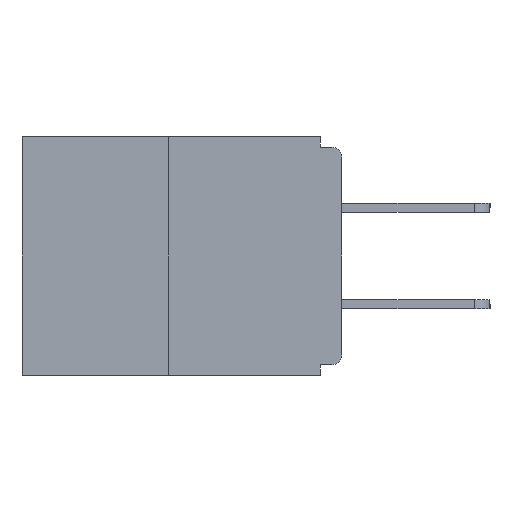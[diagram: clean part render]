
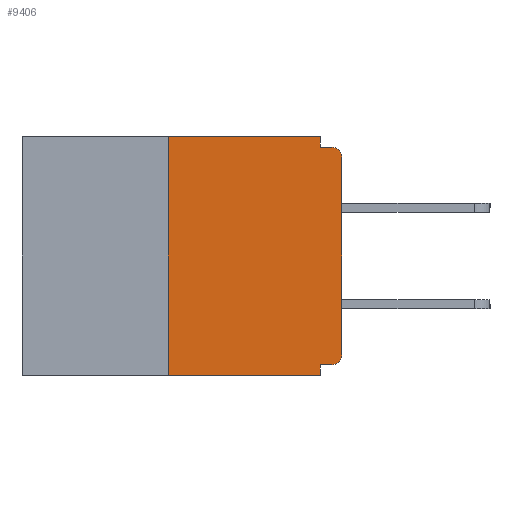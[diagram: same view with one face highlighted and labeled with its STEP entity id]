
A CAD part, left-side view. The second image highlights one B-rep face of the part: STEP entity #9406.
In plain terms, the highlighted planar face has unit normal (-1, 0, 0).
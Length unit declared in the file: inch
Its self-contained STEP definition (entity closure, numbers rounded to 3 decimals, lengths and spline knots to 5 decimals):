
#80 = VERTEX_POINT ( 'NONE', #13878 ) ;
#172 = VERTEX_POINT ( 'NONE', #8825 ) ;
#313 = CARTESIAN_POINT ( 'NONE',  ( 0., 0.015, -0.313 ) ) ;
#504 = LINE ( 'NONE', #13749, #7984 ) ;
#730 = EDGE_CURVE ( 'NONE', #14701, #11607, #9278, .T. ) ;
#771 = LINE ( 'NONE', #9872, #14488 ) ;
#1022 = VECTOR ( 'NONE', #3126, 39.37008 ) ;
#1107 = VERTEX_POINT ( 'NONE', #13405 ) ;
#1111 = AXIS2_PLACEMENT_3D ( 'NONE', #313, #15336, #6957 ) ;
#1168 = CARTESIAN_POINT ( 'NONE',  ( 0., 0., 0. ) ) ;
#1412 = CARTESIAN_POINT ( 'NONE',  ( 0., 0.015, -0.328 ) ) ;
#1575 = CARTESIAN_POINT ( 'NONE',  ( 0., 0.46, -0.343 ) ) ;
#1617 = DIRECTION ( 'NONE',  ( 1., 0., 0. ) ) ;
#1954 = ORIENTED_EDGE ( 'NONE', *, *, #13852, .F. ) ;
#2118 = EDGE_CURVE ( 'NONE', #15486, #172, #3852, .T. ) ;
#2410 = DIRECTION ( 'NONE',  ( 0., 0., 1. ) ) ;
#2470 = VECTOR ( 'NONE', #14246, 39.37008 ) ;
#3126 = DIRECTION ( 'NONE',  ( 0., 0., -1. ) ) ;
#3182 = CARTESIAN_POINT ( 'NONE',  ( 0., 0.031, 0. ) ) ;
#3269 = EDGE_CURVE ( 'NONE', #80, #11607, #504, .T. ) ;
#3852 = LINE ( 'NONE', #15900, #9210 ) ;
#4081 = VECTOR ( 'NONE', #6860, 39.37008 ) ;
#5184 = ORIENTED_EDGE ( 'NONE', *, *, #7156, .T. ) ;
#5277 = CARTESIAN_POINT ( 'NONE',  ( 0., 0.015, -0.03 ) ) ;
#6860 = DIRECTION ( 'NONE',  ( 0., -1., 0. ) ) ;
#6922 = EDGE_CURVE ( 'NONE', #14485, #11233, #11307, .T. ) ;
#6957 = DIRECTION ( 'NONE',  ( 0., 0., -1. ) ) ;
#7137 = AXIS2_PLACEMENT_3D ( 'NONE', #8317, #1617, #16765 ) ;
#7156 = EDGE_CURVE ( 'NONE', #1107, #14701, #9352, .T. ) ;
#7200 = ORIENTED_EDGE ( 'NONE', *, *, #6922, .F. ) ;
#7305 = CARTESIAN_POINT ( 'NONE',  ( 0., 0.015, -0.015 ) ) ;
#7648 = CIRCLE ( 'NONE', #1111, 0.015 ) ;
#7684 = CARTESIAN_POINT ( 'NONE',  ( 0., 0.031, -0.343 ) ) ;
#7907 = DIRECTION ( 'NONE',  ( 0., 0., -1. ) ) ;
#7984 = VECTOR ( 'NONE', #8351, 39.37008 ) ;
#8054 = EDGE_CURVE ( 'NONE', #11233, #14137, #771, .T. ) ;
#8214 = EDGE_CURVE ( 'NONE', #172, #8375, #12112, .T. ) ;
#8317 = CARTESIAN_POINT ( 'NONE',  ( 0., 0.46, 0. ) ) ;
#8351 = DIRECTION ( 'NONE',  ( 0., -1., 0. ) ) ;
#8375 = VERTEX_POINT ( 'NONE', #7684 ) ;
#8595 = LINE ( 'NONE', #1575, #4081 ) ;
#8604 = DIRECTION ( 'NONE',  ( 0., -1., 0. ) ) ;
#8675 = ORIENTED_EDGE ( 'NONE', *, *, #3269, .F. ) ;
#8825 = CARTESIAN_POINT ( 'NONE',  ( 0., 0.031, -0.328 ) ) ;
#8828 = EDGE_CURVE ( 'NONE', #14485, #8375, #8595, .T. ) ;
#9210 = VECTOR ( 'NONE', #10452, 39.37008 ) ;
#9224 = DIRECTION ( 'NONE',  ( -1., 0., 0. ) ) ;
#9278 = CIRCLE ( 'NONE', #13974, 0.015 ) ;
#9352 = LINE ( 'NONE', #1168, #12998 ) ;
#9406 = ADVANCED_FACE ( 'NONE', ( #16803 ), #16652, .F. ) ;
#9797 = LINE ( 'NONE', #3182, #1022 ) ;
#9872 = CARTESIAN_POINT ( 'NONE',  ( 0., 0.46, 0. ) ) ;
#10452 = DIRECTION ( 'NONE',  ( 0., 1., 0. ) ) ;
#10947 = DIRECTION ( 'NONE',  ( 0., 0., 1. ) ) ;
#11212 = ORIENTED_EDGE ( 'NONE', *, *, #730, .T. ) ;
#11233 = VERTEX_POINT ( 'NONE', #13191 ) ;
#11307 = LINE ( 'NONE', #11829, #14946 ) ;
#11607 = VERTEX_POINT ( 'NONE', #7305 ) ;
#11829 = CARTESIAN_POINT ( 'NONE',  ( 0., 0.25, 0. ) ) ;
#11855 = ORIENTED_EDGE ( 'NONE', *, *, #8828, .T. ) ;
#12112 = LINE ( 'NONE', #14357, #2470 ) ;
#12998 = VECTOR ( 'NONE', #10947, 39.37008 ) ;
#13191 = CARTESIAN_POINT ( 'NONE',  ( 0., 0.25, 0. ) ) ;
#13405 = CARTESIAN_POINT ( 'NONE',  ( 0., 0., -0.313 ) ) ;
#13526 = EDGE_CURVE ( 'NONE', #15486, #1107, #7648, .T. ) ;
#13531 = CARTESIAN_POINT ( 'NONE',  ( 0., 0.031, 0. ) ) ;
#13749 = CARTESIAN_POINT ( 'NONE',  ( 0., 0., -0.015 ) ) ;
#13852 = EDGE_CURVE ( 'NONE', #14137, #80, #9797, .T. ) ;
#13878 = CARTESIAN_POINT ( 'NONE',  ( 0., 0.031, -0.015 ) ) ;
#13974 = AXIS2_PLACEMENT_3D ( 'NONE', #5277, #9224, #7907 ) ;
#13993 = CARTESIAN_POINT ( 'NONE',  ( 0., 0., -0.03 ) ) ;
#14137 = VERTEX_POINT ( 'NONE', #13531 ) ;
#14246 = DIRECTION ( 'NONE',  ( 0., 0., -1. ) ) ;
#14357 = CARTESIAN_POINT ( 'NONE',  ( 0., 0.031, -0.343 ) ) ;
#14485 = VERTEX_POINT ( 'NONE', #17593 ) ;
#14488 = VECTOR ( 'NONE', #8604, 39.37008 ) ;
#14667 = ORIENTED_EDGE ( 'NONE', *, *, #2118, .F. ) ;
#14701 = VERTEX_POINT ( 'NONE', #13993 ) ;
#14946 = VECTOR ( 'NONE', #2410, 39.37008 ) ;
#15336 = DIRECTION ( 'NONE',  ( -1., 0., 0. ) ) ;
#15486 = VERTEX_POINT ( 'NONE', #1412 ) ;
#15551 = EDGE_LOOP ( 'NONE', ( #16530, #7200, #11855, #16766, #14667, #17387, #5184, #11212, #8675, #1954 ) ) ;
#15900 = CARTESIAN_POINT ( 'NONE',  ( 0., 0., -0.328 ) ) ;
#16530 = ORIENTED_EDGE ( 'NONE', *, *, #8054, .F. ) ;
#16652 = PLANE ( 'NONE',  #7137 ) ;
#16765 = DIRECTION ( 'NONE',  ( 0., 0., -1. ) ) ;
#16766 = ORIENTED_EDGE ( 'NONE', *, *, #8214, .F. ) ;
#16803 = FACE_OUTER_BOUND ( 'NONE', #15551, .T. ) ;
#17387 = ORIENTED_EDGE ( 'NONE', *, *, #13526, .T. ) ;
#17593 = CARTESIAN_POINT ( 'NONE',  ( 0., 0.25, -0.343 ) ) ;
